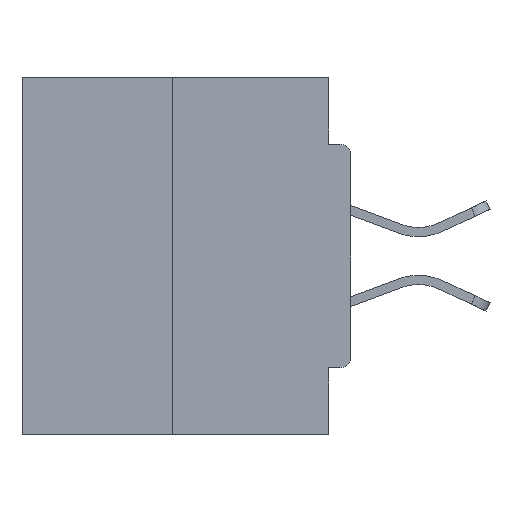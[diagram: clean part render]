
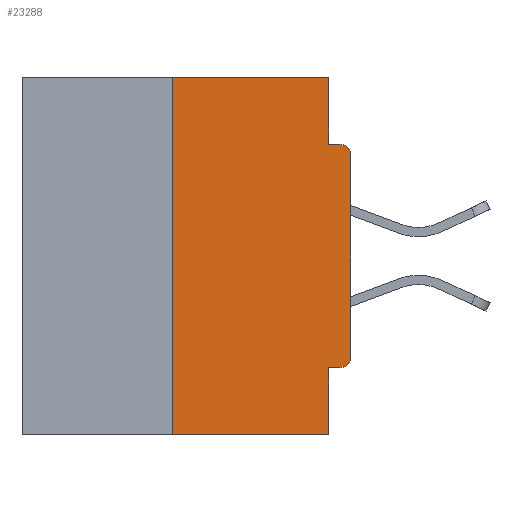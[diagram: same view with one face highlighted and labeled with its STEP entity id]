
A CAD part, left-side view. The second image highlights one B-rep face of the part: STEP entity #23288.
In plain terms, the highlighted planar face has unit normal (-1, 0, 0).
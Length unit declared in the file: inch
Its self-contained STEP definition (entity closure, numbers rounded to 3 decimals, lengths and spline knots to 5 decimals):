
#214 = VERTEX_POINT ( 'NONE', #24338 ) ;
#533 = CARTESIAN_POINT ( 'NONE',  ( 0., 0.015, -0.3915 ) ) ;
#889 = DIRECTION ( 'NONE',  ( -1., 0., 0. ) ) ;
#1049 = EDGE_CURVE ( 'NONE', #23674, #18650, #20285, .T. ) ;
#1176 = EDGE_CURVE ( 'NONE', #2993, #27672, #25942, .T. ) ;
#2063 = CIRCLE ( 'NONE', #10191, 0.015 ) ;
#2406 = ORIENTED_EDGE ( 'NONE', *, *, #1049, .F. ) ;
#2521 = VECTOR ( 'NONE', #15845, 39.37008 ) ;
#2934 = CARTESIAN_POINT ( 'NONE',  ( 0., 0., -0.1085 ) ) ;
#2993 = VERTEX_POINT ( 'NONE', #20403 ) ;
#3096 = CARTESIAN_POINT ( 'NONE',  ( 0., 0.031, 0. ) ) ;
#3115 = EDGE_CURVE ( 'NONE', #24830, #30891, #31772, .T. ) ;
#3285 = CARTESIAN_POINT ( 'NONE',  ( 0., 0., -0.4065 ) ) ;
#3344 = FACE_OUTER_BOUND ( 'NONE', #18275, .T. ) ;
#3880 = VECTOR ( 'NONE', #13163, 39.37008 ) ;
#5644 = ORIENTED_EDGE ( 'NONE', *, *, #7673, .T. ) ;
#6518 = VERTEX_POINT ( 'NONE', #2934 ) ;
#7184 = ORIENTED_EDGE ( 'NONE', *, *, #18262, .F. ) ;
#7351 = LINE ( 'NONE', #17721, #19647 ) ;
#7673 = EDGE_CURVE ( 'NONE', #6518, #22486, #2063, .T. ) ;
#8114 = CARTESIAN_POINT ( 'NONE',  ( 0., 0.46, 0. ) ) ;
#8460 = CARTESIAN_POINT ( 'NONE',  ( 0., 0.46, 0. ) ) ;
#8463 = DIRECTION ( 'NONE',  ( 0., 0., -1. ) ) ;
#9202 = ORIENTED_EDGE ( 'NONE', *, *, #26714, .F. ) ;
#9293 = ORIENTED_EDGE ( 'NONE', *, *, #3115, .F. ) ;
#10191 = AXIS2_PLACEMENT_3D ( 'NONE', #24188, #889, #21634 ) ;
#11182 = CARTESIAN_POINT ( 'NONE',  ( 0., 0.25, -0.5 ) ) ;
#11654 = ORIENTED_EDGE ( 'NONE', *, *, #20824, .F. ) ;
#13163 = DIRECTION ( 'NONE',  ( 0., 1., 0. ) ) ;
#13220 = DIRECTION ( 'NONE',  ( 1., 0., 0. ) ) ;
#13698 = EDGE_CURVE ( 'NONE', #22715, #18650, #27779, .T. ) ;
#14454 = LINE ( 'NONE', #24650, #25089 ) ;
#15554 = DIRECTION ( 'NONE',  ( 0., 0., 1. ) ) ;
#15845 = DIRECTION ( 'NONE',  ( 0., 0., -1. ) ) ;
#16271 = PLANE ( 'NONE',  #23496 ) ;
#16408 = VECTOR ( 'NONE', #8463, 39.37008 ) ;
#16461 = LINE ( 'NONE', #29377, #16408 ) ;
#16827 = DIRECTION ( 'NONE',  ( 0., -1., 0. ) ) ;
#17721 = CARTESIAN_POINT ( 'NONE',  ( 0., 0., 0. ) ) ;
#17774 = CARTESIAN_POINT ( 'NONE',  ( 0., 0.25, 0. ) ) ;
#18133 = ORIENTED_EDGE ( 'NONE', *, *, #1176, .T. ) ;
#18262 = EDGE_CURVE ( 'NONE', #22715, #24830, #25427, .T. ) ;
#18275 = EDGE_LOOP ( 'NONE', ( #9293, #7184, #29019, #2406, #9202, #18133, #26219, #5644, #25004, #11654 ) ) ;
#18650 = VERTEX_POINT ( 'NONE', #20413 ) ;
#18833 = CARTESIAN_POINT ( 'NONE',  ( 0., 0., -0.3915 ) ) ;
#19036 = DIRECTION ( 'NONE',  ( -1., 0., 0. ) ) ;
#19647 = VECTOR ( 'NONE', #22996, 39.37008 ) ;
#20285 = LINE ( 'NONE', #20618, #2521 ) ;
#20403 = CARTESIAN_POINT ( 'NONE',  ( 0., 0.015, -0.4065 ) ) ;
#20413 = CARTESIAN_POINT ( 'NONE',  ( 0., 0.031, -0.5 ) ) ;
#20618 = CARTESIAN_POINT ( 'NONE',  ( 0., 0.031, -0.5 ) ) ;
#20824 = EDGE_CURVE ( 'NONE', #30891, #214, #16461, .T. ) ;
#21539 = AXIS2_PLACEMENT_3D ( 'NONE', #533, #19036, #31665 ) ;
#21555 = DIRECTION ( 'NONE',  ( 0., -1., 0. ) ) ;
#21634 = DIRECTION ( 'NONE',  ( 0., 0., -1. ) ) ;
#22257 = EDGE_CURVE ( 'NONE', #27672, #6518, #7351, .T. ) ;
#22481 = EDGE_CURVE ( 'NONE', #214, #22486, #14454, .T. ) ;
#22486 = VERTEX_POINT ( 'NONE', #22620 ) ;
#22620 = CARTESIAN_POINT ( 'NONE',  ( 0., 0.015, -0.0935 ) ) ;
#22631 = VECTOR ( 'NONE', #30679, 39.37008 ) ;
#22715 = VERTEX_POINT ( 'NONE', #11182 ) ;
#22855 = CARTESIAN_POINT ( 'NONE',  ( 0., 0.46, -0.5 ) ) ;
#22996 = DIRECTION ( 'NONE',  ( 0., 0., 1. ) ) ;
#23288 = ADVANCED_FACE ( 'NONE', ( #3344 ), #16271, .F. ) ;
#23496 = AXIS2_PLACEMENT_3D ( 'NONE', #8114, #13220, #23599 ) ;
#23599 = DIRECTION ( 'NONE',  ( 0., 0., -1. ) ) ;
#23674 = VERTEX_POINT ( 'NONE', #29003 ) ;
#24188 = CARTESIAN_POINT ( 'NONE',  ( 0., 0.015, -0.1085 ) ) ;
#24338 = CARTESIAN_POINT ( 'NONE',  ( 0., 0.031, -0.0935 ) ) ;
#24536 = VECTOR ( 'NONE', #15554, 39.37008 ) ;
#24650 = CARTESIAN_POINT ( 'NONE',  ( 0., 0., -0.0935 ) ) ;
#24830 = VERTEX_POINT ( 'NONE', #28322 ) ;
#25004 = ORIENTED_EDGE ( 'NONE', *, *, #22481, .F. ) ;
#25089 = VECTOR ( 'NONE', #16827, 39.37008 ) ;
#25427 = LINE ( 'NONE', #17774, #24536 ) ;
#25942 = CIRCLE ( 'NONE', #21539, 0.015 ) ;
#26219 = ORIENTED_EDGE ( 'NONE', *, *, #22257, .T. ) ;
#26714 = EDGE_CURVE ( 'NONE', #2993, #23674, #28465, .T. ) ;
#27672 = VERTEX_POINT ( 'NONE', #18833 ) ;
#27779 = LINE ( 'NONE', #22855, #22631 ) ;
#28322 = CARTESIAN_POINT ( 'NONE',  ( 0., 0.25, 0. ) ) ;
#28465 = LINE ( 'NONE', #3285, #3880 ) ;
#29003 = CARTESIAN_POINT ( 'NONE',  ( 0., 0.031, -0.4065 ) ) ;
#29019 = ORIENTED_EDGE ( 'NONE', *, *, #13698, .T. ) ;
#29057 = VECTOR ( 'NONE', #21555, 39.37008 ) ;
#29377 = CARTESIAN_POINT ( 'NONE',  ( 0., 0.031, 0. ) ) ;
#30679 = DIRECTION ( 'NONE',  ( 0., -1., 0. ) ) ;
#30891 = VERTEX_POINT ( 'NONE', #3096 ) ;
#31665 = DIRECTION ( 'NONE',  ( 0., 0., -1. ) ) ;
#31772 = LINE ( 'NONE', #8460, #29057 ) ;
